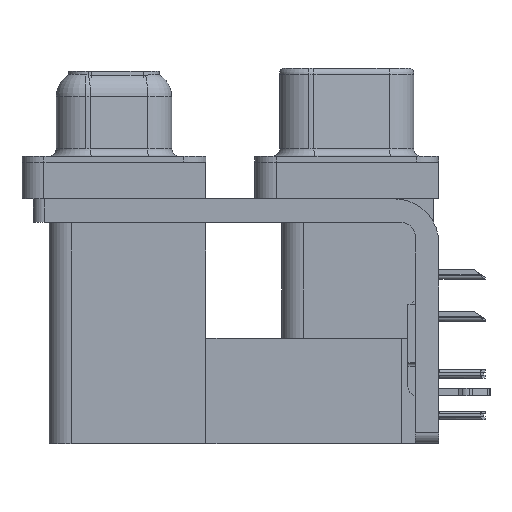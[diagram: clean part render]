
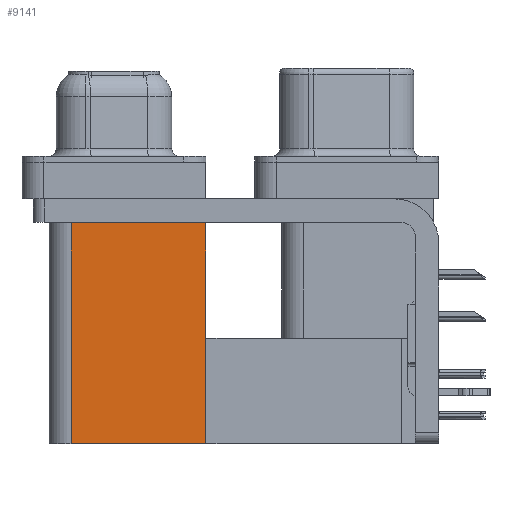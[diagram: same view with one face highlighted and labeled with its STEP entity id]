
A CAD part, left-side view. The second image highlights one B-rep face of the part: STEP entity #9141.
In plain terms, the highlighted planar face has unit normal (-1, 0, 0).
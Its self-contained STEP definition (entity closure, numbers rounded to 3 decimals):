
#239 = VECTOR ( 'NONE', #42938, 1000. ) ;
#540 = EDGE_CURVE ( 'NONE', #22119, #45939, #3206, .T. ) ;
#1098 = DIRECTION ( 'NONE',  ( 0., 1., 0. ) ) ;
#3047 = VERTEX_POINT ( 'NONE', #45852 ) ;
#3206 = LINE ( 'NONE', #37009, #4362 ) ;
#4362 = VECTOR ( 'NONE', #15870, 1000. ) ;
#4781 = DIRECTION ( 'NONE',  ( 1., 0., 0. ) ) ;
#8566 = CARTESIAN_POINT ( 'NONE',  ( 3.7, 9.6, -19.2 ) ) ;
#9141 = ADVANCED_FACE ( 'NONE', ( #35020 ), #51773, .F. ) ;
#10013 = CARTESIAN_POINT ( 'NONE',  ( 3.7, 18.8, -2.5 ) ) ;
#14139 = CARTESIAN_POINT ( 'NONE',  ( 3.7, 9.6, -19.2 ) ) ;
#14353 = EDGE_LOOP ( 'NONE', ( #46750, #19059, #32775, #39738 ) ) ;
#15870 = DIRECTION ( 'NONE',  ( 0., 1., 0. ) ) ;
#18691 = LINE ( 'NONE', #22561, #41785 ) ;
#19059 = ORIENTED_EDGE ( 'NONE', *, *, #25210, .F. ) ;
#20519 = VECTOR ( 'NONE', #1098, 1000. ) ;
#20975 = LINE ( 'NONE', #8566, #20519 ) ;
#21583 = DIRECTION ( 'NONE',  ( 0., 0., -1. ) ) ;
#22119 = VERTEX_POINT ( 'NONE', #22628 ) ;
#22395 = VERTEX_POINT ( 'NONE', #53654 ) ;
#22561 = CARTESIAN_POINT ( 'NONE',  ( 3.7, 9.6, -19.2 ) ) ;
#22628 = CARTESIAN_POINT ( 'NONE',  ( 3.7, 9.6, -2.5 ) ) ;
#25210 = EDGE_CURVE ( 'NONE', #22395, #45939, #38812, .T. ) ;
#25512 = AXIS2_PLACEMENT_3D ( 'NONE', #14139, #4781, #21583 ) ;
#30023 = EDGE_CURVE ( 'NONE', #3047, #22119, #18691, .T. ) ;
#30258 = DIRECTION ( 'NONE',  ( 0., 0., 1. ) ) ;
#32775 = ORIENTED_EDGE ( 'NONE', *, *, #42295, .F. ) ;
#34138 = CARTESIAN_POINT ( 'NONE',  ( 3.7, 18.8, -19.2 ) ) ;
#35020 = FACE_OUTER_BOUND ( 'NONE', #14353, .T. ) ;
#37009 = CARTESIAN_POINT ( 'NONE',  ( 3.7, 9.6, -2.5 ) ) ;
#38812 = LINE ( 'NONE', #34138, #239 ) ;
#39738 = ORIENTED_EDGE ( 'NONE', *, *, #30023, .T. ) ;
#41785 = VECTOR ( 'NONE', #30258, 1000. ) ;
#42295 = EDGE_CURVE ( 'NONE', #3047, #22395, #20975, .T. ) ;
#42938 = DIRECTION ( 'NONE',  ( 0., 0., 1. ) ) ;
#45852 = CARTESIAN_POINT ( 'NONE',  ( 3.7, 9.6, -19.2 ) ) ;
#45939 = VERTEX_POINT ( 'NONE', #10013 ) ;
#46750 = ORIENTED_EDGE ( 'NONE', *, *, #540, .T. ) ;
#51773 = PLANE ( 'NONE',  #25512 ) ;
#53654 = CARTESIAN_POINT ( 'NONE',  ( 3.7, 18.8, -19.2 ) ) ;
